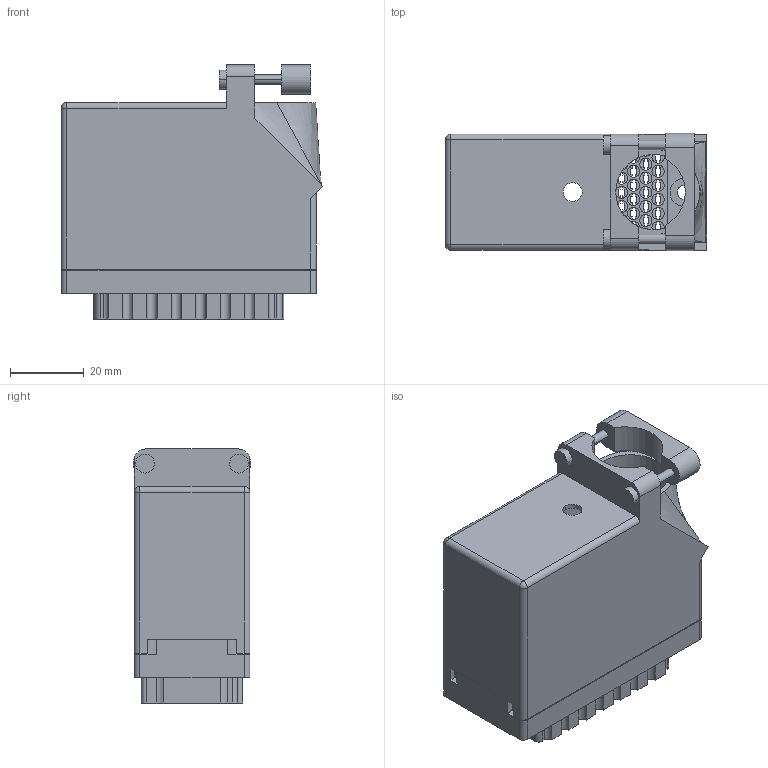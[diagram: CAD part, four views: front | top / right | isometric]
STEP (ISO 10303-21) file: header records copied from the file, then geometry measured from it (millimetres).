
FILE_DESCRIPTION (( 'STEP AP203' ), '1' );
FILE_NAME ('516-090-000-610.STEP', '2020-03-06T16:49:49', ( '' ), ( '' ), 'SwSTEP 2.0', 'SolidWorks 2016', '' );
FILE_SCHEMA (( 'CONFIG_CONTROL_DESIGN' ));
Length unit declared in the file: inch
Products named in the file (3): 516-090-000-610; 516 Part Receptacle_090; 516-230-001_Plastic - 090 Top Entry
Assembly tree (2 placements, depth 2):
  516-090-000-610
    516 Part Receptacle_090
    516-230-001_Plastic - 090 Top Entry
Bounding box: 70.83 x 31.75 x 68.73 mm (x, y, z)
Volume: 37167.3 mm3; surface area: 51597.9 mm2
Topology: 2 solids, 2 shells, 1995 faces, 5902 edges, 3930 vertices
Faces by surface type: plane 1412, cylinder 576, bspline 3, cone 2, sphere 2
Entity records: 67476 total; most frequent: CARTESIAN_POINT 11931, ORIENTED_EDGE 11800, DIRECTION 11401, EDGE_CURVE 5900, VECTOR 4385, LINE 4385, VERTEX_POINT 3930, AXIS2_PLACEMENT_3D 3508
